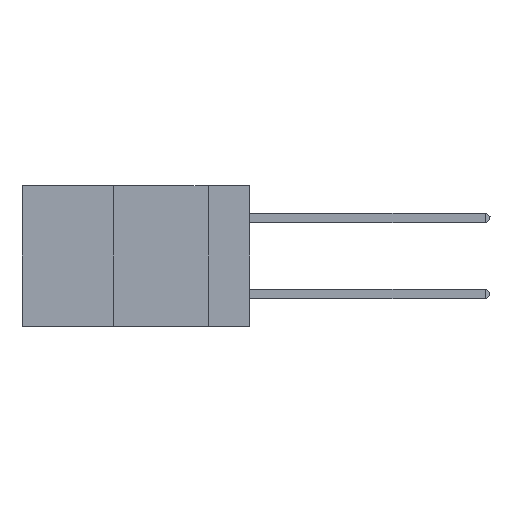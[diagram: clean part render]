
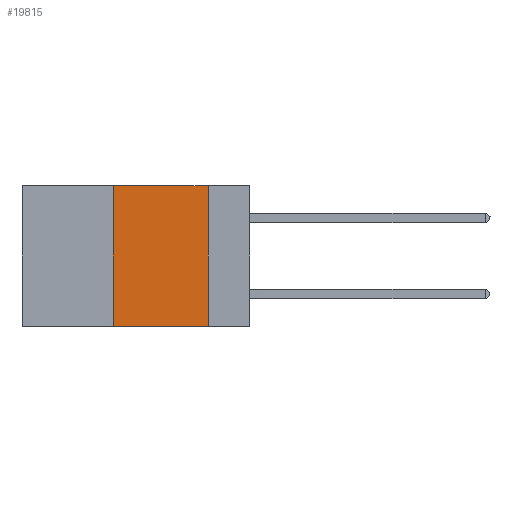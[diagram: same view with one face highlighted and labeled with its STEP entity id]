
A CAD part, left-side view. The second image highlights one B-rep face of the part: STEP entity #19815.
In plain terms, the highlighted planar face has unit normal (-1, 0, 0).
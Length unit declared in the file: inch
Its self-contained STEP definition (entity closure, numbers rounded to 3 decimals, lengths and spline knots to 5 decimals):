
#598 = CARTESIAN_POINT ( 'NONE',  ( 0., 0.6, 0. ) ) ;
#1159 = EDGE_CURVE ( 'NONE', #23626, #12170, #11897, .T. ) ;
#3769 = EDGE_LOOP ( 'NONE', ( #22321, #15204, #7326, #20511 ) ) ;
#4070 = DIRECTION ( 'NONE',  ( 0., 0., 1. ) ) ;
#6269 = DIRECTION ( 'NONE',  ( 0., -1., 0. ) ) ;
#6776 = LINE ( 'NONE', #598, #17834 ) ;
#7230 = VECTOR ( 'NONE', #15238, 39.37008 ) ;
#7326 = ORIENTED_EDGE ( 'NONE', *, *, #15700, .F. ) ;
#8189 = AXIS2_PLACEMENT_3D ( 'NONE', #23581, #18204, #8663 ) ;
#8663 = DIRECTION ( 'NONE',  ( 0., 0., -1. ) ) ;
#10575 = VECTOR ( 'NONE', #4070, 39.37008 ) ;
#10637 = CARTESIAN_POINT ( 'NONE',  ( 0., 0.36, 0. ) ) ;
#11897 = LINE ( 'NONE', #16862, #7230 ) ;
#12095 = LINE ( 'NONE', #14289, #16439 ) ;
#12170 = VERTEX_POINT ( 'NONE', #20841 ) ;
#14289 = CARTESIAN_POINT ( 'NONE',  ( 0., 0.11, 0. ) ) ;
#14387 = CARTESIAN_POINT ( 'NONE',  ( 0., 0.11, 0. ) ) ;
#14573 = EDGE_CURVE ( 'NONE', #16196, #12170, #12095, .T. ) ;
#15039 = CARTESIAN_POINT ( 'NONE',  ( 0., 0.36, 0. ) ) ;
#15204 = ORIENTED_EDGE ( 'NONE', *, *, #15955, .F. ) ;
#15238 = DIRECTION ( 'NONE',  ( 0., -1., 0. ) ) ;
#15700 = EDGE_CURVE ( 'NONE', #23626, #21064, #22498, .T. ) ;
#15955 = EDGE_CURVE ( 'NONE', #21064, #16196, #6776, .T. ) ;
#16196 = VERTEX_POINT ( 'NONE', #14387 ) ;
#16396 = PLANE ( 'NONE',  #8189 ) ;
#16439 = VECTOR ( 'NONE', #21873, 39.37008 ) ;
#16862 = CARTESIAN_POINT ( 'NONE',  ( 0., 0.6, -0.37 ) ) ;
#17834 = VECTOR ( 'NONE', #6269, 39.37008 ) ;
#18204 = DIRECTION ( 'NONE',  ( 1., 0., 0. ) ) ;
#18982 = CARTESIAN_POINT ( 'NONE',  ( 0., 0.36, -0.37 ) ) ;
#19071 = FACE_OUTER_BOUND ( 'NONE', #3769, .T. ) ;
#19815 = ADVANCED_FACE ( 'NONE', ( #19071 ), #16396, .F. ) ;
#20511 = ORIENTED_EDGE ( 'NONE', *, *, #1159, .T. ) ;
#20841 = CARTESIAN_POINT ( 'NONE',  ( 0., 0.11, -0.37 ) ) ;
#21064 = VERTEX_POINT ( 'NONE', #10637 ) ;
#21873 = DIRECTION ( 'NONE',  ( 0., 0., -1. ) ) ;
#22321 = ORIENTED_EDGE ( 'NONE', *, *, #14573, .F. ) ;
#22498 = LINE ( 'NONE', #15039, #10575 ) ;
#23581 = CARTESIAN_POINT ( 'NONE',  ( 0., 0.6, 0. ) ) ;
#23626 = VERTEX_POINT ( 'NONE', #18982 ) ;
